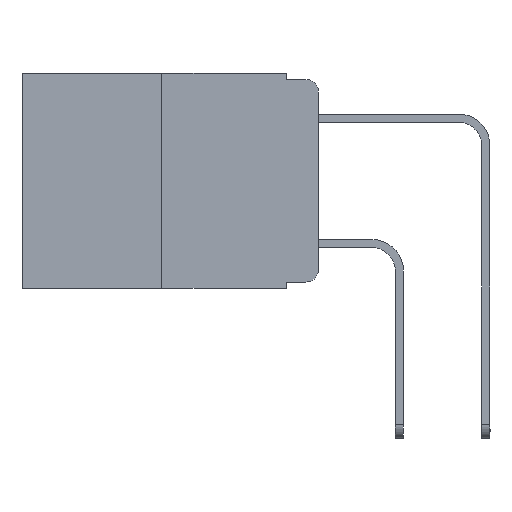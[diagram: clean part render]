
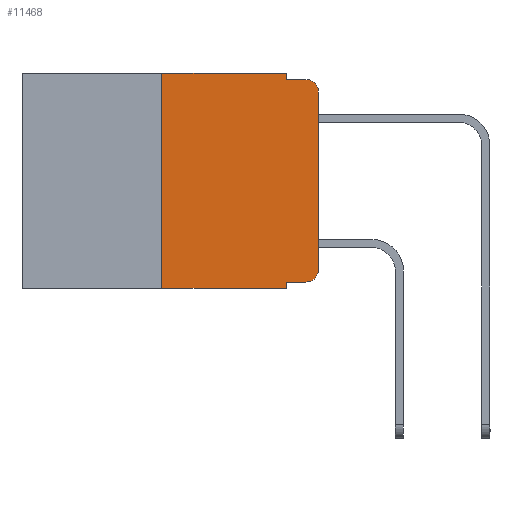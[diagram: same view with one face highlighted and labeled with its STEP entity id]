
A CAD part, left-side view. The second image highlights one B-rep face of the part: STEP entity #11468.
In plain terms, the highlighted planar face has unit normal (-1, 0, 0).
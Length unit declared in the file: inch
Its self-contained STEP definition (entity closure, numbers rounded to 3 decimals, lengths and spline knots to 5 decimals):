
#200 = CARTESIAN_POINT ( 'NONE',  ( 0., 0.051, 0. ) ) ;
#1276 = LINE ( 'NONE', #25989, #7845 ) ;
#1835 = ORIENTED_EDGE ( 'NONE', *, *, #17257, .T. ) ;
#2676 = CARTESIAN_POINT ( 'NONE',  ( 0., 0.02, -0.313 ) ) ;
#2703 = VERTEX_POINT ( 'NONE', #3565 ) ;
#3083 = CARTESIAN_POINT ( 'NONE',  ( 0., 0.02, -0.03 ) ) ;
#3493 = VERTEX_POINT ( 'NONE', #5568 ) ;
#3565 = CARTESIAN_POINT ( 'NONE',  ( 0., 0.051, -0.343 ) ) ;
#3696 = CARTESIAN_POINT ( 'NONE',  ( 0., 0.25, 0. ) ) ;
#3982 = VERTEX_POINT ( 'NONE', #11061 ) ;
#4282 = CARTESIAN_POINT ( 'NONE',  ( 0., 0.051, 0. ) ) ;
#4368 = LINE ( 'NONE', #200, #6979 ) ;
#4879 = LINE ( 'NONE', #4282, #19140 ) ;
#4978 = DIRECTION ( 'NONE',  ( 0., 0., -1. ) ) ;
#5119 = LINE ( 'NONE', #19601, #10014 ) ;
#5153 = VECTOR ( 'NONE', #25551, 39.37008 ) ;
#5455 = EDGE_CURVE ( 'NONE', #26042, #7519, #9665, .T. ) ;
#5568 = CARTESIAN_POINT ( 'NONE',  ( 0., 0.051, 0. ) ) ;
#5590 = VERTEX_POINT ( 'NONE', #21703 ) ;
#5623 = ORIENTED_EDGE ( 'NONE', *, *, #14985, .T. ) ;
#6399 = DIRECTION ( 'NONE',  ( 0., -1., 0. ) ) ;
#6426 = ORIENTED_EDGE ( 'NONE', *, *, #5455, .F. ) ;
#6469 = DIRECTION ( 'NONE',  ( 0., 0., -1. ) ) ;
#6558 = VECTOR ( 'NONE', #16671, 39.37008 ) ;
#6979 = VECTOR ( 'NONE', #14944, 39.37008 ) ;
#7108 = LINE ( 'NONE', #23740, #5153 ) ;
#7206 = DIRECTION ( 'NONE',  ( 0., 0., 1. ) ) ;
#7279 = LINE ( 'NONE', #8591, #10878 ) ;
#7519 = VERTEX_POINT ( 'NONE', #3696 ) ;
#7770 = AXIS2_PLACEMENT_3D ( 'NONE', #3083, #11223, #13284 ) ;
#7845 = VECTOR ( 'NONE', #19586, 39.37008 ) ;
#8089 = CARTESIAN_POINT ( 'NONE',  ( 0., 0.25, -0.343 ) ) ;
#8212 = EDGE_CURVE ( 'NONE', #11970, #3982, #26445, .T. ) ;
#8567 = DIRECTION ( 'NONE',  ( 0., 0., 1. ) ) ;
#8591 = CARTESIAN_POINT ( 'NONE',  ( 0., 0.473, -0.343 ) ) ;
#8655 = CARTESIAN_POINT ( 'NONE',  ( 0., 0.25, 0. ) ) ;
#9175 = ORIENTED_EDGE ( 'NONE', *, *, #25569, .F. ) ;
#9325 = EDGE_CURVE ( 'NONE', #22365, #24314, #15976, .T. ) ;
#9431 = CARTESIAN_POINT ( 'NONE',  ( 0., 0.051, -0.01 ) ) ;
#9490 = DIRECTION ( 'NONE',  ( 0., 0., -1. ) ) ;
#9554 = EDGE_CURVE ( 'NONE', #9643, #24314, #1276, .T. ) ;
#9643 = VERTEX_POINT ( 'NONE', #9431 ) ;
#9665 = LINE ( 'NONE', #8655, #20372 ) ;
#10014 = VECTOR ( 'NONE', #7206, 39.37008 ) ;
#10220 = AXIS2_PLACEMENT_3D ( 'NONE', #2676, #17225, #4978 ) ;
#10878 = VECTOR ( 'NONE', #6399, 39.37008 ) ;
#11061 = CARTESIAN_POINT ( 'NONE',  ( 0., 0., -0.313 ) ) ;
#11223 = DIRECTION ( 'NONE',  ( -1., 0., 0. ) ) ;
#11468 = ADVANCED_FACE ( 'NONE', ( #16457 ), #21907, .F. ) ;
#11970 = VERTEX_POINT ( 'NONE', #17594 ) ;
#12220 = CARTESIAN_POINT ( 'NONE',  ( 0., 0., -0.03 ) ) ;
#13284 = DIRECTION ( 'NONE',  ( 0., 0., -1. ) ) ;
#13646 = DIRECTION ( 'NONE',  ( 1., 0., 0. ) ) ;
#13746 = ORIENTED_EDGE ( 'NONE', *, *, #8212, .T. ) ;
#13994 = ORIENTED_EDGE ( 'NONE', *, *, #23505, .T. ) ;
#14944 = DIRECTION ( 'NONE',  ( 0., 0., -1. ) ) ;
#14985 = EDGE_CURVE ( 'NONE', #5590, #11970, #26045, .T. ) ;
#15800 = CARTESIAN_POINT ( 'NONE',  ( 0., 0.473, 0. ) ) ;
#15976 = CIRCLE ( 'NONE', #7770, 0.02 ) ;
#16457 = FACE_OUTER_BOUND ( 'NONE', #19969, .T. ) ;
#16671 = DIRECTION ( 'NONE',  ( 0., -1., 0. ) ) ;
#17225 = DIRECTION ( 'NONE',  ( -1., 0., 0. ) ) ;
#17257 = EDGE_CURVE ( 'NONE', #3982, #22365, #5119, .T. ) ;
#17594 = CARTESIAN_POINT ( 'NONE',  ( 0., 0.02, -0.333 ) ) ;
#18983 = ORIENTED_EDGE ( 'NONE', *, *, #19441, .F. ) ;
#19140 = VECTOR ( 'NONE', #6469, 39.37008 ) ;
#19441 = EDGE_CURVE ( 'NONE', #3493, #9643, #4879, .T. ) ;
#19586 = DIRECTION ( 'NONE',  ( 0., -1., 0. ) ) ;
#19601 = CARTESIAN_POINT ( 'NONE',  ( 0., 0., 0. ) ) ;
#19969 = EDGE_LOOP ( 'NONE', ( #1835, #23692, #21202, #18983, #9175, #6426, #13994, #19992, #5623, #13746 ) ) ;
#19992 = ORIENTED_EDGE ( 'NONE', *, *, #23037, .F. ) ;
#20372 = VECTOR ( 'NONE', #8567, 39.37008 ) ;
#21202 = ORIENTED_EDGE ( 'NONE', *, *, #9554, .F. ) ;
#21703 = CARTESIAN_POINT ( 'NONE',  ( 0., 0.051, -0.333 ) ) ;
#21907 = PLANE ( 'NONE',  #24500 ) ;
#22365 = VERTEX_POINT ( 'NONE', #12220 ) ;
#23037 = EDGE_CURVE ( 'NONE', #5590, #2703, #4368, .T. ) ;
#23505 = EDGE_CURVE ( 'NONE', #26042, #2703, #7279, .T. ) ;
#23692 = ORIENTED_EDGE ( 'NONE', *, *, #9325, .T. ) ;
#23740 = CARTESIAN_POINT ( 'NONE',  ( 0., 0.473, 0. ) ) ;
#24314 = VERTEX_POINT ( 'NONE', #25700 ) ;
#24500 = AXIS2_PLACEMENT_3D ( 'NONE', #15800, #13646, #9490 ) ;
#25043 = CARTESIAN_POINT ( 'NONE',  ( 0., 0.051, -0.333 ) ) ;
#25551 = DIRECTION ( 'NONE',  ( 0., -1., 0. ) ) ;
#25569 = EDGE_CURVE ( 'NONE', #7519, #3493, #7108, .T. ) ;
#25700 = CARTESIAN_POINT ( 'NONE',  ( 0., 0.02, -0.01 ) ) ;
#25989 = CARTESIAN_POINT ( 'NONE',  ( 0., 0.051, -0.01 ) ) ;
#26042 = VERTEX_POINT ( 'NONE', #8089 ) ;
#26045 = LINE ( 'NONE', #25043, #6558 ) ;
#26445 = CIRCLE ( 'NONE', #10220, 0.02 ) ;
